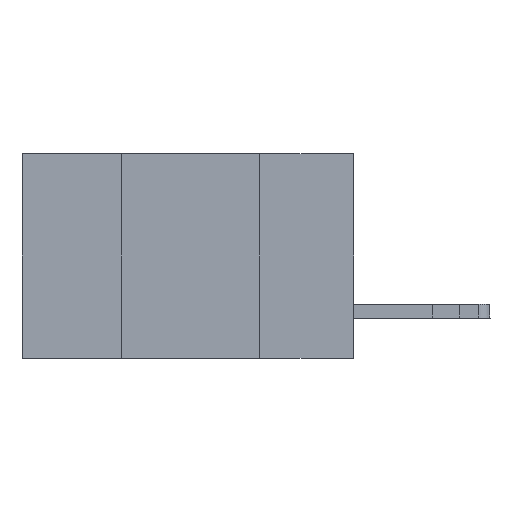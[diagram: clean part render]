
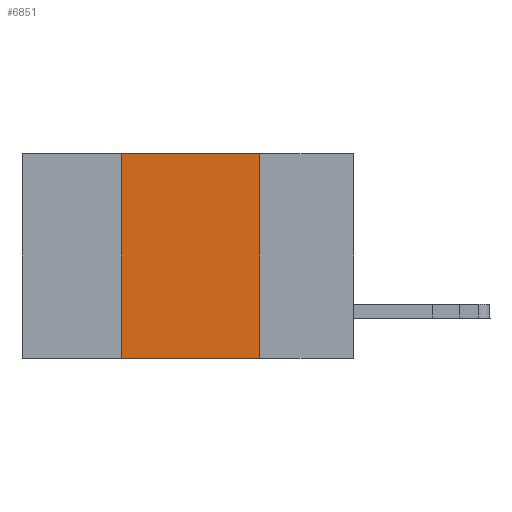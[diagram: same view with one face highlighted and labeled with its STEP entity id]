
A CAD part, left-side view. The second image highlights one B-rep face of the part: STEP entity #6851.
In plain terms, the highlighted planar face has unit normal (-1, 0, 0).
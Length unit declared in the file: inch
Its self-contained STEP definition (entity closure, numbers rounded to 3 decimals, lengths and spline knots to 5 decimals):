
#1200 = CARTESIAN_POINT ( 'NONE',  ( 0., 0.42, 0. ) ) ;
#1546 = DIRECTION ( 'NONE',  ( 1., 0., 0. ) ) ;
#1563 = CARTESIAN_POINT ( 'NONE',  ( 0., 0.42, 0. ) ) ;
#2453 = CARTESIAN_POINT ( 'NONE',  ( 0., 0.6, -0.37 ) ) ;
#3143 = CARTESIAN_POINT ( 'NONE',  ( 0., 0.17, 0. ) ) ;
#3167 = DIRECTION ( 'NONE',  ( 0., -1., 0. ) ) ;
#4855 = VERTEX_POINT ( 'NONE', #15192 ) ;
#6310 = VECTOR ( 'NONE', #16436, 39.37008 ) ;
#6555 = VERTEX_POINT ( 'NONE', #7790 ) ;
#6666 = VERTEX_POINT ( 'NONE', #1200 ) ;
#6851 = ADVANCED_FACE ( 'NONE', ( #16317 ), #7030, .F. ) ;
#6996 = EDGE_CURVE ( 'NONE', #6666, #6555, #14285, .T. ) ;
#7030 = PLANE ( 'NONE',  #11086 ) ;
#7386 = ORIENTED_EDGE ( 'NONE', *, *, #6996, .F. ) ;
#7670 = EDGE_CURVE ( 'NONE', #6555, #14619, #15681, .T. ) ;
#7790 = CARTESIAN_POINT ( 'NONE',  ( 0., 0.17, 0. ) ) ;
#8010 = VECTOR ( 'NONE', #3167, 39.37008 ) ;
#8328 = EDGE_CURVE ( 'NONE', #4855, #6666, #13455, .T. ) ;
#9005 = EDGE_LOOP ( 'NONE', ( #16713, #7386, #11359, #14892 ) ) ;
#9373 = VECTOR ( 'NONE', #10602, 39.37008 ) ;
#9925 = DIRECTION ( 'NONE',  ( 0., 0., -1. ) ) ;
#10602 = DIRECTION ( 'NONE',  ( 0., -1., 0. ) ) ;
#10696 = EDGE_CURVE ( 'NONE', #4855, #14619, #12953, .T. ) ;
#11065 = DIRECTION ( 'NONE',  ( 0., 0., -1. ) ) ;
#11086 = AXIS2_PLACEMENT_3D ( 'NONE', #12355, #1546, #11065 ) ;
#11294 = CARTESIAN_POINT ( 'NONE',  ( 0., 0.6, 0. ) ) ;
#11359 = ORIENTED_EDGE ( 'NONE', *, *, #8328, .F. ) ;
#12355 = CARTESIAN_POINT ( 'NONE',  ( 0., 0.6, 0. ) ) ;
#12953 = LINE ( 'NONE', #2453, #9373 ) ;
#13455 = LINE ( 'NONE', #1563, #6310 ) ;
#14285 = LINE ( 'NONE', #11294, #8010 ) ;
#14372 = CARTESIAN_POINT ( 'NONE',  ( 0., 0.17, -0.37 ) ) ;
#14619 = VERTEX_POINT ( 'NONE', #14372 ) ;
#14892 = ORIENTED_EDGE ( 'NONE', *, *, #10696, .T. ) ;
#15192 = CARTESIAN_POINT ( 'NONE',  ( 0., 0.42, -0.37 ) ) ;
#15276 = VECTOR ( 'NONE', #9925, 39.37008 ) ;
#15681 = LINE ( 'NONE', #3143, #15276 ) ;
#16317 = FACE_OUTER_BOUND ( 'NONE', #9005, .T. ) ;
#16436 = DIRECTION ( 'NONE',  ( 0., 0., 1. ) ) ;
#16713 = ORIENTED_EDGE ( 'NONE', *, *, #7670, .F. ) ;
